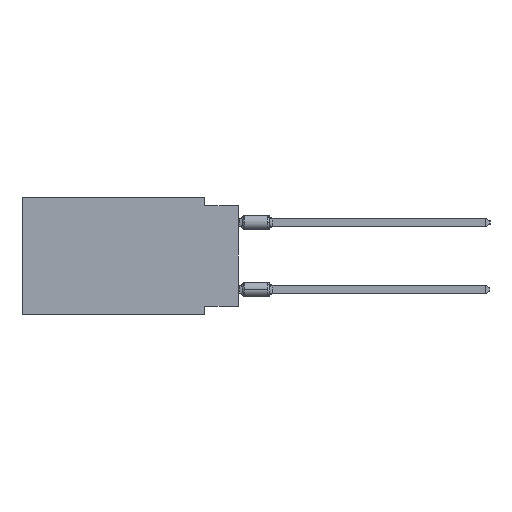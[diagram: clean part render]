
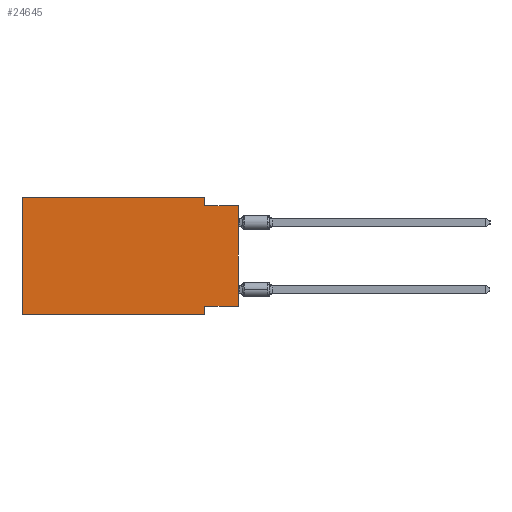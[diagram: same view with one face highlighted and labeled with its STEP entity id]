
A CAD part, left-side view. The second image highlights one B-rep face of the part: STEP entity #24645.
In plain terms, the highlighted planar face has unit normal (-1, 0, 0).
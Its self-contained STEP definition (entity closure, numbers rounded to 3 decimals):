
#73 = LINE ( 'NONE', #15131, #3784 ) ;
#149 = ORIENTED_EDGE ( 'NONE', *, *, #38298, .T. ) ;
#1184 = DIRECTION ( 'NONE',  ( 0., 0., -1. ) ) ;
#1308 = CARTESIAN_POINT ( 'NONE',  ( 0., 2.54, -8.89 ) ) ;
#1782 = FACE_OUTER_BOUND ( 'NONE', #18103, .T. ) ;
#2125 = CARTESIAN_POINT ( 'NONE',  ( 0., 0., -8.255 ) ) ;
#2416 = EDGE_CURVE ( 'NONE', #13102, #26532, #37623, .T. ) ;
#3220 = EDGE_CURVE ( 'NONE', #33620, #10866, #34054, .T. ) ;
#3301 = LINE ( 'NONE', #36880, #24904 ) ;
#3433 = EDGE_CURVE ( 'NONE', #10866, #13102, #17139, .T. ) ;
#3442 = CARTESIAN_POINT ( 'NONE',  ( 0., 0., -0.635 ) ) ;
#3470 = DIRECTION ( 'NONE',  ( 0., 0., 1. ) ) ;
#3681 = VECTOR ( 'NONE', #3470, 1000. ) ;
#3784 = VECTOR ( 'NONE', #8310, 1000. ) ;
#4378 = ORIENTED_EDGE ( 'NONE', *, *, #2416, .F. ) ;
#6038 = VERTEX_POINT ( 'NONE', #26877 ) ;
#6272 = EDGE_CURVE ( 'NONE', #6038, #12437, #23232, .T. ) ;
#7115 = ORIENTED_EDGE ( 'NONE', *, *, #31185, .F. ) ;
#7274 = CARTESIAN_POINT ( 'NONE',  ( 0., 16.383, 0. ) ) ;
#8310 = DIRECTION ( 'NONE',  ( 0., 0., 1. ) ) ;
#8532 = LINE ( 'NONE', #2125, #27754 ) ;
#9884 = CARTESIAN_POINT ( 'NONE',  ( 0., 0., -8.255 ) ) ;
#10866 = VERTEX_POINT ( 'NONE', #19052 ) ;
#11628 = CARTESIAN_POINT ( 'NONE',  ( 0., 16.383, 0. ) ) ;
#12437 = VERTEX_POINT ( 'NONE', #20256 ) ;
#13102 = VERTEX_POINT ( 'NONE', #35855 ) ;
#13458 = ORIENTED_EDGE ( 'NONE', *, *, #3433, .F. ) ;
#13529 = DIRECTION ( 'NONE',  ( 0., -1., 0. ) ) ;
#14049 = DIRECTION ( 'NONE',  ( 1., 0., 0. ) ) ;
#15131 = CARTESIAN_POINT ( 'NONE',  ( 0., 0., 0. ) ) ;
#17139 = LINE ( 'NONE', #23184, #32540 ) ;
#17487 = VERTEX_POINT ( 'NONE', #20323 ) ;
#18103 = EDGE_LOOP ( 'NONE', ( #149, #4378, #13458, #22925, #26423, #28571, #26763, #7115 ) ) ;
#19052 = CARTESIAN_POINT ( 'NONE',  ( 0., 2.54, 0. ) ) ;
#19307 = EDGE_CURVE ( 'NONE', #17487, #33620, #25775, .T. ) ;
#20256 = CARTESIAN_POINT ( 'NONE',  ( 0., 2.54, -8.89 ) ) ;
#20323 = CARTESIAN_POINT ( 'NONE',  ( 0., 16.383, -8.89 ) ) ;
#22925 = ORIENTED_EDGE ( 'NONE', *, *, #3220, .F. ) ;
#23184 = CARTESIAN_POINT ( 'NONE',  ( 0., 2.54, 0. ) ) ;
#23232 = LINE ( 'NONE', #1308, #26480 ) ;
#24112 = VECTOR ( 'NONE', #37437, 1000. ) ;
#24166 = VECTOR ( 'NONE', #13529, 1000. ) ;
#24645 = ADVANCED_FACE ( 'NONE', ( #1782 ), #25732, .F. ) ;
#24904 = VECTOR ( 'NONE', #36691, 1000. ) ;
#25732 = PLANE ( 'NONE',  #33162 ) ;
#25775 = LINE ( 'NONE', #7274, #3681 ) ;
#26423 = ORIENTED_EDGE ( 'NONE', *, *, #19307, .F. ) ;
#26480 = VECTOR ( 'NONE', #35506, 1000. ) ;
#26532 = VERTEX_POINT ( 'NONE', #26634 ) ;
#26634 = CARTESIAN_POINT ( 'NONE',  ( 0., 0., -0.635 ) ) ;
#26763 = ORIENTED_EDGE ( 'NONE', *, *, #6272, .F. ) ;
#26877 = CARTESIAN_POINT ( 'NONE',  ( 0., 2.54, -8.255 ) ) ;
#27754 = VECTOR ( 'NONE', #32469, 1000. ) ;
#28571 = ORIENTED_EDGE ( 'NONE', *, *, #36974, .T. ) ;
#28724 = CARTESIAN_POINT ( 'NONE',  ( 0., 16.383, 0. ) ) ;
#31185 = EDGE_CURVE ( 'NONE', #37166, #6038, #8532, .T. ) ;
#32469 = DIRECTION ( 'NONE',  ( 0., 1., 0. ) ) ;
#32540 = VECTOR ( 'NONE', #35460, 1000. ) ;
#33162 = AXIS2_PLACEMENT_3D ( 'NONE', #28724, #14049, #1184 ) ;
#33620 = VERTEX_POINT ( 'NONE', #11628 ) ;
#34054 = LINE ( 'NONE', #34651, #24166 ) ;
#34651 = CARTESIAN_POINT ( 'NONE',  ( 0., 16.383, 0. ) ) ;
#35460 = DIRECTION ( 'NONE',  ( 0., 0., -1. ) ) ;
#35506 = DIRECTION ( 'NONE',  ( 0., 0., -1. ) ) ;
#35855 = CARTESIAN_POINT ( 'NONE',  ( 0., 2.54, -0.635 ) ) ;
#36691 = DIRECTION ( 'NONE',  ( 0., -1., 0. ) ) ;
#36880 = CARTESIAN_POINT ( 'NONE',  ( 0., 16.383, -8.89 ) ) ;
#36974 = EDGE_CURVE ( 'NONE', #17487, #12437, #3301, .T. ) ;
#37166 = VERTEX_POINT ( 'NONE', #9884 ) ;
#37437 = DIRECTION ( 'NONE',  ( 0., -1., 0. ) ) ;
#37623 = LINE ( 'NONE', #3442, #24112 ) ;
#38298 = EDGE_CURVE ( 'NONE', #37166, #26532, #73, .T. ) ;
